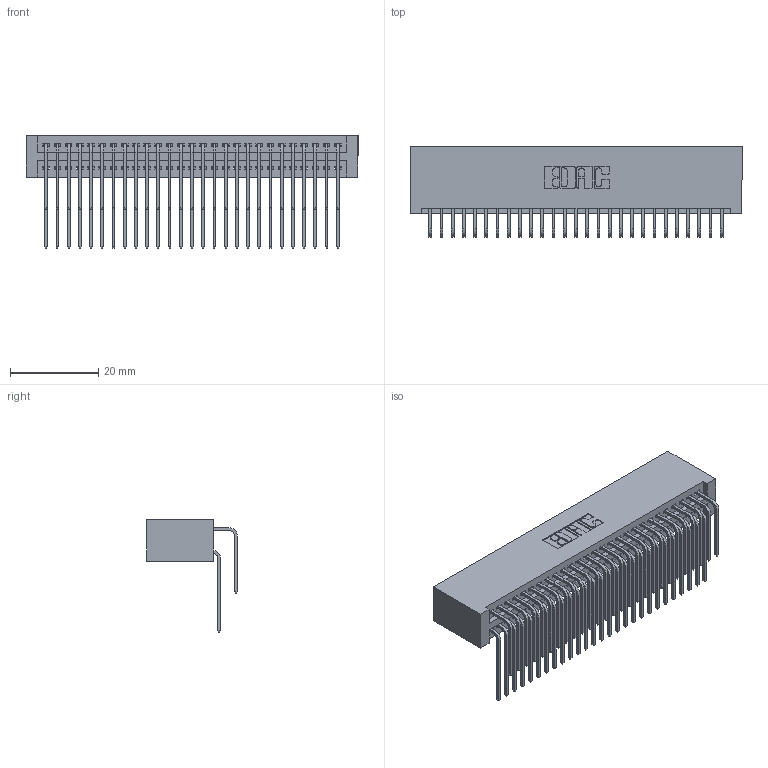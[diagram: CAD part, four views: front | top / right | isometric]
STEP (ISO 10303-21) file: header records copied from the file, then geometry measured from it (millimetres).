
FILE_DESCRIPTION (( 'STEP AP203' ), '1' );
FILE_NAME ('345-054-559-201.STEP', '2019-10-29T20:08:34', ( '' ), ( '' ), 'SwSTEP 2.0', 'SolidWorks 2016', '' );
FILE_SCHEMA (( 'CONFIG_CONTROL_DESIGN' ));
Length unit declared in the file: inch
Products named in the file (4): 345-292-001_559 Tail - 2; 345-054-559-201; 345-292-001_558 559 Tail - 1; 345 Part_No Mounting Lugs
Assembly tree (55 placements, depth 2):
  345-054-559-201
    345 Part_No Mounting Lugs
    345-292-001_558 559 Tail - 1  x27
    345-292-001_559 Tail - 2  x27
Bounding box: 75.18 x 20.56 x 25.53 mm (x, y, z)
Volume: 8091.6 mm3; surface area: 13438.4 mm2
Topology: 55 solids, 55 shells, 2926 faces, 8687 edges, 5718 vertices
Faces by surface type: plane 1966, cylinder 960
Entity records: 24579 total; most frequent: CARTESIAN_POINT 4179, ORIENTED_EDGE 4062, DIRECTION 3671, EDGE_CURVE 2031, LINE 1759, VECTOR 1759, VERTEX_POINT 1350, AXIS2_PLACEMENT_3D 956
